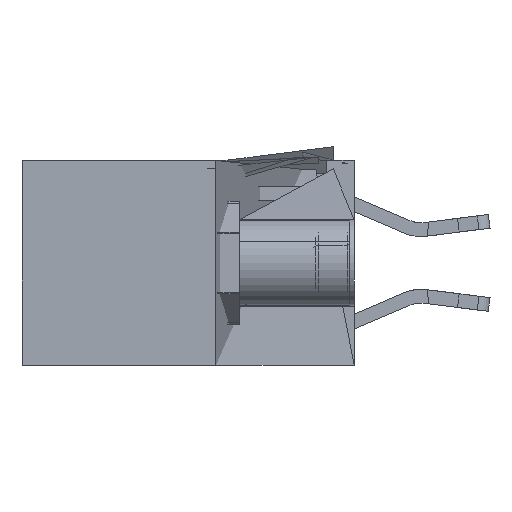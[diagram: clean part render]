
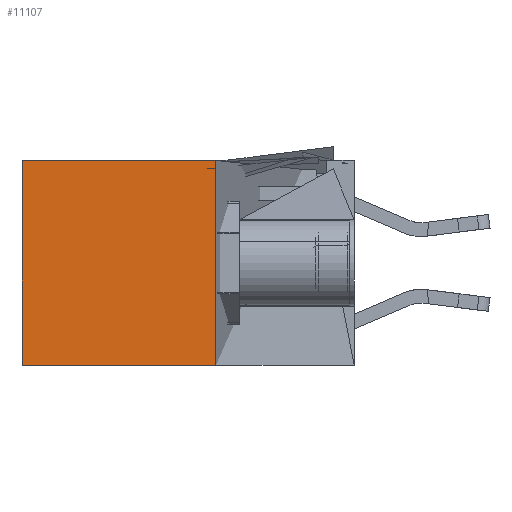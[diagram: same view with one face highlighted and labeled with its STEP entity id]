
A CAD part, left-side view. The second image highlights one B-rep face of the part: STEP entity #11107.
In plain terms, the highlighted face is planar.
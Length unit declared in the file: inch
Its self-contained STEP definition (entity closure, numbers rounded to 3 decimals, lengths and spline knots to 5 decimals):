
#59 = ORIENTED_EDGE ( 'NONE', *, *, #6426, .T. ) ;
#207 = EDGE_CURVE ( 'NONE', #21377, #15622, #28464, .T. ) ;
#293 = ORIENTED_EDGE ( 'NONE', *, *, #26546, .F. ) ;
#2555 = DIRECTION ( 'NONE',  ( 1., 0., 0. ) ) ;
#3174 = DIRECTION ( 'NONE',  ( 0., 0., -1. ) ) ;
#3738 = CARTESIAN_POINT ( 'NONE',  ( 0.2625, 0.25, 0. ) ) ;
#5063 = CARTESIAN_POINT ( 'NONE',  ( 0.2625, 0.25, -0.37 ) ) ;
#5143 = CARTESIAN_POINT ( 'NONE',  ( 0.2625, 0.6, -0.37 ) ) ;
#6426 = EDGE_CURVE ( 'NONE', #11598, #15622, #14770, .T. ) ;
#6664 = PLANE ( 'NONE',  #28786 ) ;
#6933 = EDGE_CURVE ( 'NONE', #21578, #11598, #19269, .T. ) ;
#7436 = VECTOR ( 'NONE', #21513, 39.37008 ) ;
#10161 = DIRECTION ( 'NONE',  ( 0., 1., 0. ) ) ;
#10476 = DIRECTION ( 'NONE',  ( 0., 1., 0. ) ) ;
#11107 = ADVANCED_FACE ( 'NONE', ( #18097 ), #6664, .F. ) ;
#11598 = VERTEX_POINT ( 'NONE', #15295 ) ;
#12528 = VECTOR ( 'NONE', #10161, 39.37008 ) ;
#12730 = VECTOR ( 'NONE', #10476, 39.37008 ) ;
#12807 = CARTESIAN_POINT ( 'NONE',  ( 0.2625, 0.25, 0. ) ) ;
#14057 = EDGE_LOOP ( 'NONE', ( #59, #21141, #293, #23698 ) ) ;
#14770 = LINE ( 'NONE', #23701, #7436 ) ;
#15295 = CARTESIAN_POINT ( 'NONE',  ( 0.2625, 0.6, 0. ) ) ;
#15617 = DIRECTION ( 'NONE',  ( 0., 0., -1. ) ) ;
#15622 = VERTEX_POINT ( 'NONE', #5143 ) ;
#18097 = FACE_OUTER_BOUND ( 'NONE', #14057, .T. ) ;
#18571 = LINE ( 'NONE', #27367, #21568 ) ;
#19269 = LINE ( 'NONE', #3738, #12730 ) ;
#21141 = ORIENTED_EDGE ( 'NONE', *, *, #207, .F. ) ;
#21377 = VERTEX_POINT ( 'NONE', #26001 ) ;
#21513 = DIRECTION ( 'NONE',  ( 0., 0., -1. ) ) ;
#21568 = VECTOR ( 'NONE', #3174, 39.37008 ) ;
#21578 = VERTEX_POINT ( 'NONE', #12807 ) ;
#22343 = CARTESIAN_POINT ( 'NONE',  ( 0.2625, 0.25, 0. ) ) ;
#23698 = ORIENTED_EDGE ( 'NONE', *, *, #6933, .T. ) ;
#23701 = CARTESIAN_POINT ( 'NONE',  ( 0.2625, 0.6, 0. ) ) ;
#26001 = CARTESIAN_POINT ( 'NONE',  ( 0.2625, 0.25, -0.37 ) ) ;
#26546 = EDGE_CURVE ( 'NONE', #21578, #21377, #18571, .T. ) ;
#27367 = CARTESIAN_POINT ( 'NONE',  ( 0.2625, 0.25, 0. ) ) ;
#28464 = LINE ( 'NONE', #5063, #12528 ) ;
#28786 = AXIS2_PLACEMENT_3D ( 'NONE', #22343, #2555, #15617 ) ;
